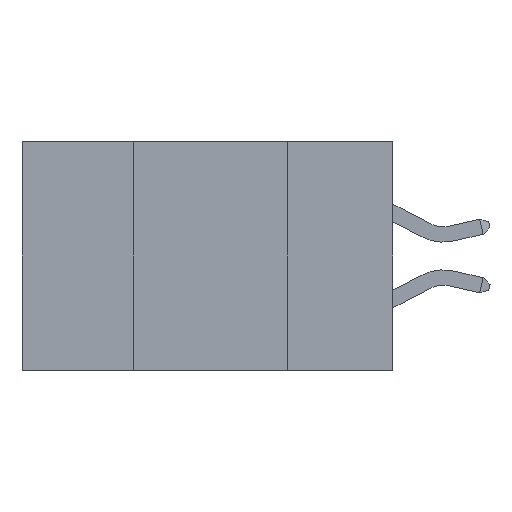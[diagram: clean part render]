
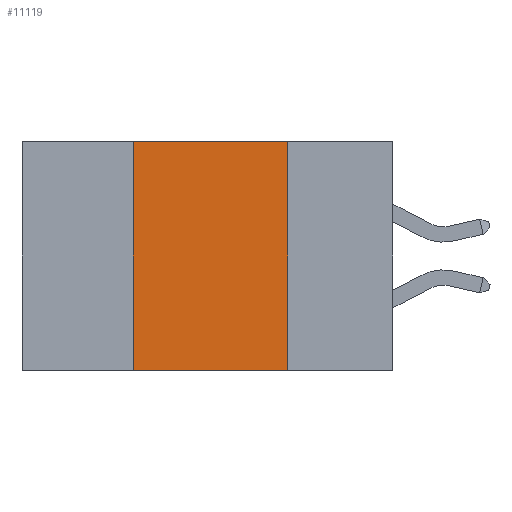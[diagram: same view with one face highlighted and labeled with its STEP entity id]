
A CAD part, left-side view. The second image highlights one B-rep face of the part: STEP entity #11119.
In plain terms, the highlighted planar face has unit normal (-1, 0, 0).
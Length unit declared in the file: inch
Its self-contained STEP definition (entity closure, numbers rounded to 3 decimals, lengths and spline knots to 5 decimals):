
#417 = EDGE_CURVE ( 'NONE', #9819, #6831, #676, .T. ) ;
#676 = LINE ( 'NONE', #2622, #3328 ) ;
#1026 = EDGE_LOOP ( 'NONE', ( #3339, #9767, #13173, #7139 ) ) ;
#1184 = EDGE_CURVE ( 'NONE', #3078, #6831, #9555, .T. ) ;
#1295 = DIRECTION ( 'NONE',  ( 0., -1., 0. ) ) ;
#1317 = CARTESIAN_POINT ( 'NONE',  ( 0., 0.6, 0. ) ) ;
#1460 = CARTESIAN_POINT ( 'NONE',  ( 0., 0.42, -0.37 ) ) ;
#1676 = CARTESIAN_POINT ( 'NONE',  ( 0., 0.6, -0.37 ) ) ;
#2046 = DIRECTION ( 'NONE',  ( 1., 0., 0. ) ) ;
#2271 = LINE ( 'NONE', #4772, #11845 ) ;
#2622 = CARTESIAN_POINT ( 'NONE',  ( 0., 0.17, 0. ) ) ;
#2650 = DIRECTION ( 'NONE',  ( 0., -1., 0. ) ) ;
#3078 = VERTEX_POINT ( 'NONE', #1460 ) ;
#3328 = VECTOR ( 'NONE', #6987, 39.37008 ) ;
#3338 = LINE ( 'NONE', #1317, #15485 ) ;
#3339 = ORIENTED_EDGE ( 'NONE', *, *, #417, .F. ) ;
#4772 = CARTESIAN_POINT ( 'NONE',  ( 0., 0.42, 0. ) ) ;
#4851 = EDGE_CURVE ( 'NONE', #3078, #6021, #2271, .T. ) ;
#6021 = VERTEX_POINT ( 'NONE', #7626 ) ;
#6831 = VERTEX_POINT ( 'NONE', #6922 ) ;
#6922 = CARTESIAN_POINT ( 'NONE',  ( 0., 0.17, -0.37 ) ) ;
#6987 = DIRECTION ( 'NONE',  ( 0., 0., -1. ) ) ;
#7139 = ORIENTED_EDGE ( 'NONE', *, *, #1184, .T. ) ;
#7626 = CARTESIAN_POINT ( 'NONE',  ( 0., 0.42, 0. ) ) ;
#7818 = EDGE_CURVE ( 'NONE', #6021, #9819, #3338, .T. ) ;
#8236 = FACE_OUTER_BOUND ( 'NONE', #1026, .T. ) ;
#9360 = CARTESIAN_POINT ( 'NONE',  ( 0., 0.6, 0. ) ) ;
#9555 = LINE ( 'NONE', #1676, #15638 ) ;
#9767 = ORIENTED_EDGE ( 'NONE', *, *, #7818, .F. ) ;
#9819 = VERTEX_POINT ( 'NONE', #12419 ) ;
#10553 = DIRECTION ( 'NONE',  ( 0., 0., -1. ) ) ;
#11119 = ADVANCED_FACE ( 'NONE', ( #8236 ), #15076, .F. ) ;
#11845 = VECTOR ( 'NONE', #14157, 39.37008 ) ;
#12419 = CARTESIAN_POINT ( 'NONE',  ( 0., 0.17, 0. ) ) ;
#13173 = ORIENTED_EDGE ( 'NONE', *, *, #4851, .F. ) ;
#14157 = DIRECTION ( 'NONE',  ( 0., 0., 1. ) ) ;
#15007 = AXIS2_PLACEMENT_3D ( 'NONE', #9360, #2046, #10553 ) ;
#15076 = PLANE ( 'NONE',  #15007 ) ;
#15485 = VECTOR ( 'NONE', #2650, 39.37008 ) ;
#15638 = VECTOR ( 'NONE', #1295, 39.37008 ) ;
